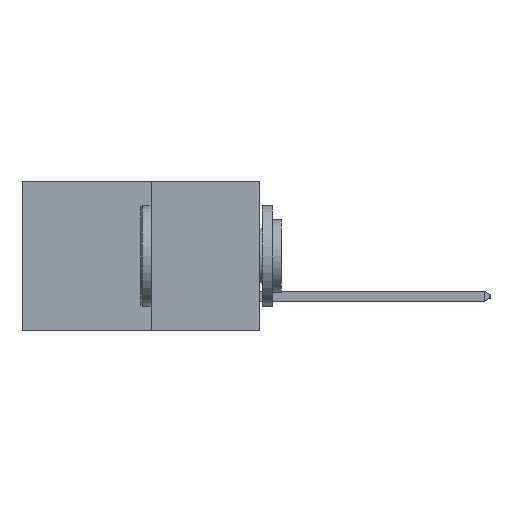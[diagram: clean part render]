
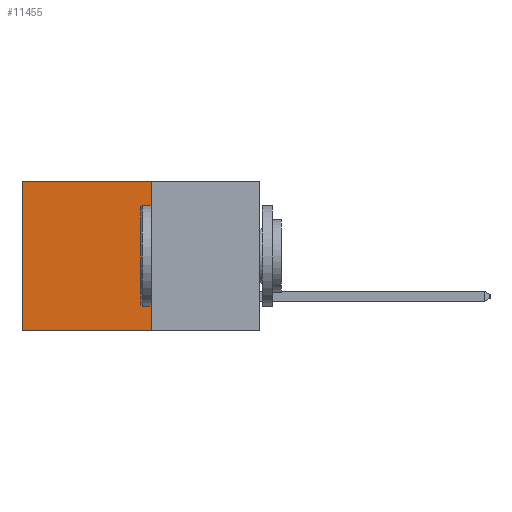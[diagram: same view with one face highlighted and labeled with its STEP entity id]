
A CAD part, left-side view. The second image highlights one B-rep face of the part: STEP entity #11455.
In plain terms, the highlighted planar face has unit normal (-1, 0, 0).
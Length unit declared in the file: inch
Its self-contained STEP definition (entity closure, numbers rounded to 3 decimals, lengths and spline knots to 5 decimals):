
#284 = EDGE_CURVE ( 'NONE', #6129, #6275, #14894, .T. ) ;
#572 = CARTESIAN_POINT ( 'NONE',  ( 0.277, 0.59, -0.37 ) ) ;
#693 = CARTESIAN_POINT ( 'NONE',  ( 0.277, 0.59, 0. ) ) ;
#1110 = CARTESIAN_POINT ( 'NONE',  ( 0.277, 0.27, -0.37 ) ) ;
#1305 = FACE_OUTER_BOUND ( 'NONE', #3388, .T. ) ;
#1749 = VECTOR ( 'NONE', #20478, 39.37008 ) ;
#3223 = LINE ( 'NONE', #18073, #11376 ) ;
#3388 = EDGE_LOOP ( 'NONE', ( #8400, #12419, #6417, #13297 ) ) ;
#3961 = AXIS2_PLACEMENT_3D ( 'NONE', #4762, #20920, #11313 ) ;
#4762 = CARTESIAN_POINT ( 'NONE',  ( 0.277, 0.27, -0.37 ) ) ;
#5046 = VERTEX_POINT ( 'NONE', #18735 ) ;
#5284 = EDGE_CURVE ( 'NONE', #12589, #6275, #19005, .T. ) ;
#6129 = VERTEX_POINT ( 'NONE', #693 ) ;
#6275 = VERTEX_POINT ( 'NONE', #11747 ) ;
#6417 = ORIENTED_EDGE ( 'NONE', *, *, #7819, .F. ) ;
#6779 = DIRECTION ( 'NONE',  ( 0., 1., 0. ) ) ;
#7819 = EDGE_CURVE ( 'NONE', #5046, #12589, #12307, .T. ) ;
#8400 = ORIENTED_EDGE ( 'NONE', *, *, #284, .T. ) ;
#11313 = DIRECTION ( 'NONE',  ( 0., 0., -1. ) ) ;
#11376 = VECTOR ( 'NONE', #6779, 39.37008 ) ;
#11455 = ADVANCED_FACE ( 'NONE', ( #1305 ), #19339, .F. ) ;
#11747 = CARTESIAN_POINT ( 'NONE',  ( 0.277, 0.59, -0.37 ) ) ;
#12307 = LINE ( 'NONE', #1110, #20375 ) ;
#12419 = ORIENTED_EDGE ( 'NONE', *, *, #5284, .F. ) ;
#12589 = VERTEX_POINT ( 'NONE', #17722 ) ;
#13297 = ORIENTED_EDGE ( 'NONE', *, *, #20034, .T. ) ;
#14894 = LINE ( 'NONE', #572, #15898 ) ;
#15724 = DIRECTION ( 'NONE',  ( 0., 0., -1. ) ) ;
#15898 = VECTOR ( 'NONE', #17004, 39.37008 ) ;
#16570 = CARTESIAN_POINT ( 'NONE',  ( 0.277, 0.27, -0.37 ) ) ;
#17004 = DIRECTION ( 'NONE',  ( 0., 0., -1. ) ) ;
#17722 = CARTESIAN_POINT ( 'NONE',  ( 0.277, 0.27, -0.37 ) ) ;
#18073 = CARTESIAN_POINT ( 'NONE',  ( 0.277, 0.27, 0. ) ) ;
#18735 = CARTESIAN_POINT ( 'NONE',  ( 0.277, 0.27, 0. ) ) ;
#19005 = LINE ( 'NONE', #16570, #1749 ) ;
#19339 = PLANE ( 'NONE',  #3961 ) ;
#20034 = EDGE_CURVE ( 'NONE', #5046, #6129, #3223, .T. ) ;
#20375 = VECTOR ( 'NONE', #15724, 39.37008 ) ;
#20478 = DIRECTION ( 'NONE',  ( 0., 1., 0. ) ) ;
#20920 = DIRECTION ( 'NONE',  ( 1., 0., 0. ) ) ;
